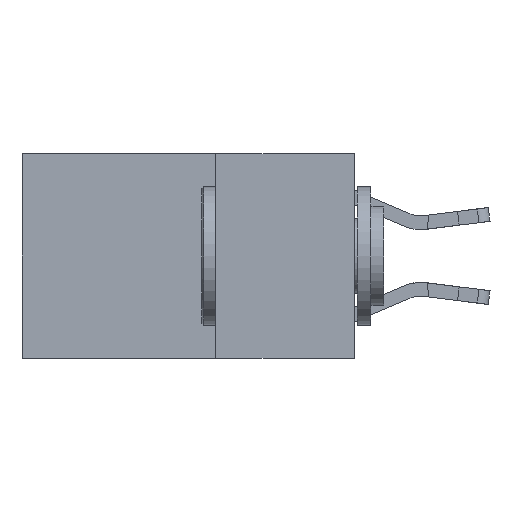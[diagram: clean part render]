
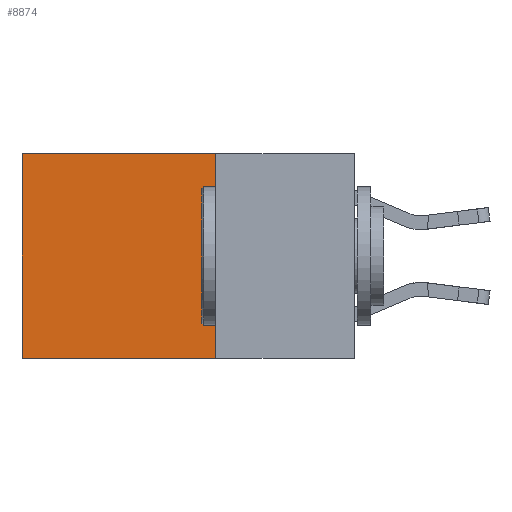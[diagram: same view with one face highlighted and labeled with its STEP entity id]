
A CAD part, left-side view. The second image highlights one B-rep face of the part: STEP entity #8874.
In plain terms, the highlighted planar face has unit normal (-1, 0, 0).
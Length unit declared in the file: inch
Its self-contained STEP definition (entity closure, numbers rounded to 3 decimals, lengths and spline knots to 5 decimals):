
#781 = DIRECTION ( 'NONE',  ( 1., 0., 0. ) ) ;
#938 = EDGE_CURVE ( 'NONE', #18798, #15492, #18471, .T. ) ;
#991 = CARTESIAN_POINT ( 'NONE',  ( 0.2625, 0.6, 0. ) ) ;
#1660 = CARTESIAN_POINT ( 'NONE',  ( 0.2625, 0.25, 0. ) ) ;
#3843 = CARTESIAN_POINT ( 'NONE',  ( 0.2625, 0.25, -0.37 ) ) ;
#4211 = VERTEX_POINT ( 'NONE', #3843 ) ;
#4801 = DIRECTION ( 'NONE',  ( 0., 1., 0. ) ) ;
#4924 = EDGE_LOOP ( 'NONE', ( #19876, #6192, #8754, #21535 ) ) ;
#6192 = ORIENTED_EDGE ( 'NONE', *, *, #12637, .F. ) ;
#6760 = PLANE ( 'NONE',  #22761 ) ;
#6987 = VECTOR ( 'NONE', #18602, 39.37008 ) ;
#7461 = EDGE_CURVE ( 'NONE', #19711, #18798, #15596, .T. ) ;
#8363 = FACE_OUTER_BOUND ( 'NONE', #4924, .T. ) ;
#8754 = ORIENTED_EDGE ( 'NONE', *, *, #13463, .F. ) ;
#8874 = ADVANCED_FACE ( 'NONE', ( #8363 ), #6760, .F. ) ;
#8888 = LINE ( 'NONE', #1660, #11524 ) ;
#9253 = VECTOR ( 'NONE', #4801, 39.37008 ) ;
#9949 = CARTESIAN_POINT ( 'NONE',  ( 0.2625, 0.25, 0. ) ) ;
#11524 = VECTOR ( 'NONE', #21967, 39.37008 ) ;
#12637 = EDGE_CURVE ( 'NONE', #4211, #15492, #20803, .T. ) ;
#13463 = EDGE_CURVE ( 'NONE', #19711, #4211, #8888, .T. ) ;
#14231 = CARTESIAN_POINT ( 'NONE',  ( 0.2625, 0.25, 0. ) ) ;
#15492 = VERTEX_POINT ( 'NONE', #23749 ) ;
#15596 = LINE ( 'NONE', #9949, #9253 ) ;
#16425 = CARTESIAN_POINT ( 'NONE',  ( 0.2625, 0.6, 0. ) ) ;
#17054 = CARTESIAN_POINT ( 'NONE',  ( 0.2625, 0.25, 0. ) ) ;
#18471 = LINE ( 'NONE', #16425, #6987 ) ;
#18602 = DIRECTION ( 'NONE',  ( 0., 0., -1. ) ) ;
#18798 = VERTEX_POINT ( 'NONE', #991 ) ;
#19484 = DIRECTION ( 'NONE',  ( 0., 0., -1. ) ) ;
#19711 = VERTEX_POINT ( 'NONE', #17054 ) ;
#19876 = ORIENTED_EDGE ( 'NONE', *, *, #938, .T. ) ;
#20803 = LINE ( 'NONE', #22875, #24004 ) ;
#21535 = ORIENTED_EDGE ( 'NONE', *, *, #7461, .T. ) ;
#21967 = DIRECTION ( 'NONE',  ( 0., 0., -1. ) ) ;
#22754 = DIRECTION ( 'NONE',  ( 0., 1., 0. ) ) ;
#22761 = AXIS2_PLACEMENT_3D ( 'NONE', #14231, #781, #19484 ) ;
#22875 = CARTESIAN_POINT ( 'NONE',  ( 0.2625, 0.25, -0.37 ) ) ;
#23749 = CARTESIAN_POINT ( 'NONE',  ( 0.2625, 0.6, -0.37 ) ) ;
#24004 = VECTOR ( 'NONE', #22754, 39.37008 ) ;
